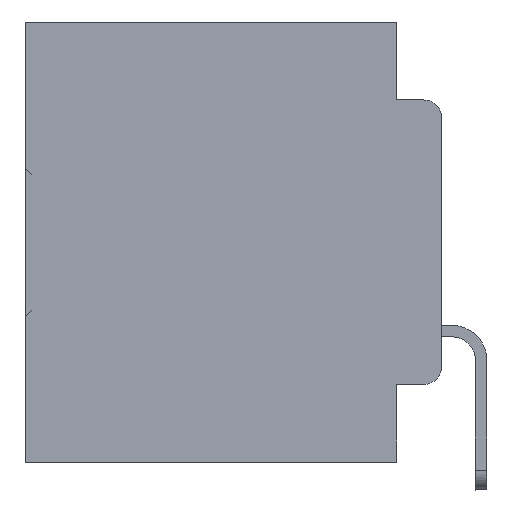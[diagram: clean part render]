
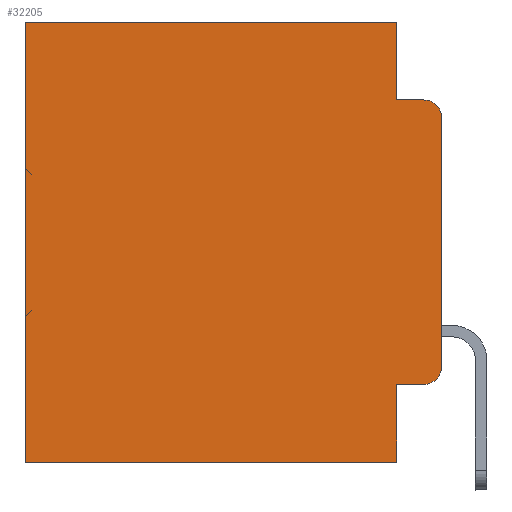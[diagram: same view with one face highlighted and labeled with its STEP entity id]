
A CAD part, left-side view. The second image highlights one B-rep face of the part: STEP entity #32205.
In plain terms, the highlighted planar face has unit normal (-1, 0, 0).
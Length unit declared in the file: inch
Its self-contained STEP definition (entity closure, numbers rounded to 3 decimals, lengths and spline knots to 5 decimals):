
#181 = ORIENTED_EDGE ( 'NONE', *, *, #33246, .T. ) ;
#350 = CARTESIAN_POINT ( 'NONE',  ( 0.298, 0.051, -0.0885 ) ) ;
#585 = CARTESIAN_POINT ( 'NONE',  ( 0.298, 0.473, -0.5 ) ) ;
#1938 = CARTESIAN_POINT ( 'NONE',  ( 0.298, 0.051, -0.0885 ) ) ;
#2297 = VECTOR ( 'NONE', #33445, 39.37008 ) ;
#2380 = ORIENTED_EDGE ( 'NONE', *, *, #25808, .T. ) ;
#2495 = EDGE_LOOP ( 'NONE', ( #35316, #181, #32342, #4215, #29399, #2380, #13563, #26129, #20125, #18918 ) ) ;
#2530 = CARTESIAN_POINT ( 'NONE',  ( 0.298, 0., 0. ) ) ;
#3123 = CARTESIAN_POINT ( 'NONE',  ( 0.298, 0.02, -0.4115 ) ) ;
#3162 = EDGE_CURVE ( 'NONE', #13598, #11919, #19119, .T. ) ;
#4215 = ORIENTED_EDGE ( 'NONE', *, *, #11333, .F. ) ;
#4368 = VERTEX_POINT ( 'NONE', #24933 ) ;
#5369 = FACE_OUTER_BOUND ( 'NONE', #2495, .T. ) ;
#5760 = CARTESIAN_POINT ( 'NONE',  ( 0.298, 0., -0.3915 ) ) ;
#6107 = AXIS2_PLACEMENT_3D ( 'NONE', #25854, #19758, #23089 ) ;
#6800 = CARTESIAN_POINT ( 'NONE',  ( 0.298, 0.051, 0. ) ) ;
#7319 = DIRECTION ( 'NONE',  ( 0., -1., 0. ) ) ;
#7325 = DIRECTION ( 'NONE',  ( 0., 1., 0. ) ) ;
#7989 = PLANE ( 'NONE',  #30335 ) ;
#8186 = CARTESIAN_POINT ( 'NONE',  ( 0.298, 0.051, -0.4115 ) ) ;
#8275 = LINE ( 'NONE', #27891, #14156 ) ;
#8966 = LINE ( 'NONE', #20256, #23029 ) ;
#9058 = EDGE_CURVE ( 'NONE', #31352, #4368, #16414, .T. ) ;
#9902 = VECTOR ( 'NONE', #7319, 39.37008 ) ;
#11333 = EDGE_CURVE ( 'NONE', #34305, #23148, #8275, .T. ) ;
#11391 = EDGE_CURVE ( 'NONE', #16778, #11919, #31206, .T. ) ;
#11594 = DIRECTION ( 'NONE',  ( 0., 0., -1. ) ) ;
#11919 = VERTEX_POINT ( 'NONE', #5760 ) ;
#11991 = LINE ( 'NONE', #34536, #29720 ) ;
#12005 = AXIS2_PLACEMENT_3D ( 'NONE', #31007, #25832, #14377 ) ;
#12421 = VECTOR ( 'NONE', #7325, 39.37008 ) ;
#13047 = CARTESIAN_POINT ( 'NONE',  ( 0.298, 0.02, -0.0885 ) ) ;
#13222 = VERTEX_POINT ( 'NONE', #585 ) ;
#13260 = LINE ( 'NONE', #1938, #9902 ) ;
#13374 = CARTESIAN_POINT ( 'NONE',  ( 0.298, 0., 0. ) ) ;
#13427 = CARTESIAN_POINT ( 'NONE',  ( 0.298, 0., -0.1085 ) ) ;
#13563 = ORIENTED_EDGE ( 'NONE', *, *, #27373, .F. ) ;
#13598 = VERTEX_POINT ( 'NONE', #3123 ) ;
#14036 = EDGE_CURVE ( 'NONE', #34305, #32439, #11991, .T. ) ;
#14156 = VECTOR ( 'NONE', #36208, 39.37008 ) ;
#14377 = DIRECTION ( 'NONE',  ( 0., 0., -1. ) ) ;
#15325 = VERTEX_POINT ( 'NONE', #13047 ) ;
#16414 = LINE ( 'NONE', #22868, #35254 ) ;
#16778 = VERTEX_POINT ( 'NONE', #13427 ) ;
#16880 = CARTESIAN_POINT ( 'NONE',  ( 0.298, 0.473, 0. ) ) ;
#18918 = ORIENTED_EDGE ( 'NONE', *, *, #3162, .T. ) ;
#19119 = CIRCLE ( 'NONE', #6107, 0.02 ) ;
#19673 = CIRCLE ( 'NONE', #12005, 0.02 ) ;
#19758 = DIRECTION ( 'NONE',  ( -1., 0., 0. ) ) ;
#20125 = ORIENTED_EDGE ( 'NONE', *, *, #26030, .T. ) ;
#20256 = CARTESIAN_POINT ( 'NONE',  ( 0.298, 0.473, 0. ) ) ;
#20314 = DIRECTION ( 'NONE',  ( 0., 1., 0. ) ) ;
#22442 = LINE ( 'NONE', #8186, #26549 ) ;
#22868 = CARTESIAN_POINT ( 'NONE',  ( 0.298, 0.051, 0. ) ) ;
#23029 = VECTOR ( 'NONE', #31529, 39.37008 ) ;
#23089 = DIRECTION ( 'NONE',  ( 0., 0., -1. ) ) ;
#23148 = VERTEX_POINT ( 'NONE', #350 ) ;
#24163 = LINE ( 'NONE', #32671, #12421 ) ;
#24644 = DIRECTION ( 'NONE',  ( 0., 0., -1. ) ) ;
#24933 = CARTESIAN_POINT ( 'NONE',  ( 0.298, 0.051, -0.5 ) ) ;
#25428 = EDGE_CURVE ( 'NONE', #23148, #15325, #13260, .T. ) ;
#25808 = EDGE_CURVE ( 'NONE', #32439, #13222, #8966, .T. ) ;
#25832 = DIRECTION ( 'NONE',  ( -1., 0., 0. ) ) ;
#25854 = CARTESIAN_POINT ( 'NONE',  ( 0.298, 0.02, -0.3915 ) ) ;
#26030 = EDGE_CURVE ( 'NONE', #31352, #13598, #22442, .T. ) ;
#26129 = ORIENTED_EDGE ( 'NONE', *, *, #9058, .F. ) ;
#26549 = VECTOR ( 'NONE', #27448, 39.37008 ) ;
#26814 = CARTESIAN_POINT ( 'NONE',  ( 0.298, 0.051, -0.4115 ) ) ;
#27373 = EDGE_CURVE ( 'NONE', #4368, #13222, #24163, .T. ) ;
#27448 = DIRECTION ( 'NONE',  ( 0., -1., 0. ) ) ;
#27891 = CARTESIAN_POINT ( 'NONE',  ( 0.298, 0.051, 0. ) ) ;
#27957 = DIRECTION ( 'NONE',  ( 1., 0., 0. ) ) ;
#29399 = ORIENTED_EDGE ( 'NONE', *, *, #14036, .T. ) ;
#29720 = VECTOR ( 'NONE', #20314, 39.37008 ) ;
#30335 = AXIS2_PLACEMENT_3D ( 'NONE', #13374, #27957, #24644 ) ;
#31007 = CARTESIAN_POINT ( 'NONE',  ( 0.298, 0.02, -0.1085 ) ) ;
#31206 = LINE ( 'NONE', #2530, #2297 ) ;
#31352 = VERTEX_POINT ( 'NONE', #26814 ) ;
#31529 = DIRECTION ( 'NONE',  ( 0., 0., -1. ) ) ;
#32205 = ADVANCED_FACE ( 'NONE', ( #5369 ), #7989, .F. ) ;
#32342 = ORIENTED_EDGE ( 'NONE', *, *, #25428, .F. ) ;
#32439 = VERTEX_POINT ( 'NONE', #16880 ) ;
#32671 = CARTESIAN_POINT ( 'NONE',  ( 0.298, 0., -0.5 ) ) ;
#33246 = EDGE_CURVE ( 'NONE', #16778, #15325, #19673, .T. ) ;
#33445 = DIRECTION ( 'NONE',  ( 0., 0., -1. ) ) ;
#34305 = VERTEX_POINT ( 'NONE', #6800 ) ;
#34536 = CARTESIAN_POINT ( 'NONE',  ( 0.298, 0., 0. ) ) ;
#35254 = VECTOR ( 'NONE', #11594, 39.37008 ) ;
#35316 = ORIENTED_EDGE ( 'NONE', *, *, #11391, .F. ) ;
#36208 = DIRECTION ( 'NONE',  ( 0., 0., -1. ) ) ;
